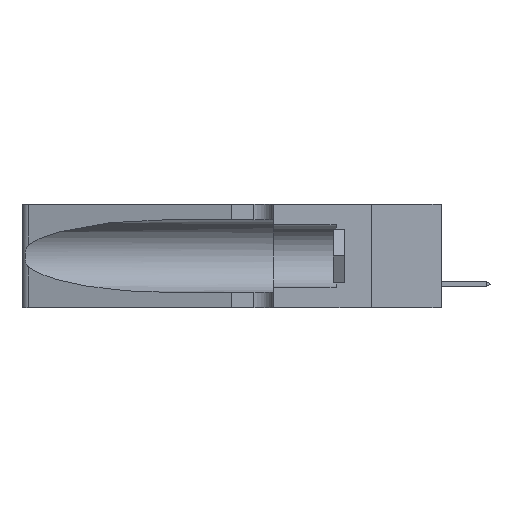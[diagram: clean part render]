
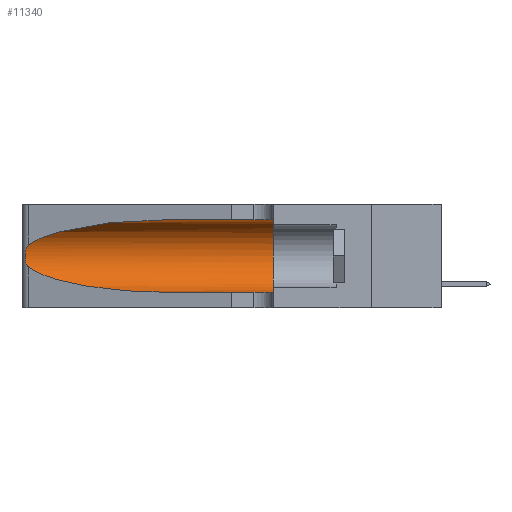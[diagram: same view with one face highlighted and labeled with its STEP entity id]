
A CAD part, left-side view. The second image highlights one B-rep face of the part: STEP entity #11340.
In plain terms, the highlighted cylindrical face has radius 3.308 mm (diameter 6.617 mm), a partial arc.
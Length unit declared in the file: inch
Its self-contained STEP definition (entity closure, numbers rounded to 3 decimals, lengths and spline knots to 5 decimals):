
#604 = EDGE_CURVE ( 'NONE', #4491, #828, #35944, .T. ) ;
#828 = VERTEX_POINT ( 'NONE', #34601 ) ;
#1053 = DIRECTION ( 'NONE',  ( 0., 0., 1. ) ) ;
#1105 = DIRECTION ( 'NONE',  ( 0., -1., 0. ) ) ;
#1410 = CARTESIAN_POINT ( 'NONE',  ( 0.1305, 0.35, 0.31525 ) ) ;
#1831 = CARTESIAN_POINT ( 'NONE',  ( 0.25487, 1.22718, 0.22369 ) ) ;
#1986 = CARTESIAN_POINT ( 'NONE',  ( 0.2373, 1.15595, 0.08982 ) ) ;
#2128 = ORIENTED_EDGE ( 'NONE', *, *, #12219, .F. ) ;
#2251 = EDGE_LOOP ( 'NONE', ( #20262, #12538, #23843, #12944, #31784, #2128 ) ) ;
#2801 = VERTEX_POINT ( 'NONE', #34864 ) ;
#3267 = CYLINDRICAL_SURFACE ( 'NONE', #34637, 0.13025 ) ;
#3283 = CARTESIAN_POINT ( 'NONE',  ( 0.25487, 1.22718, 0.22369 ) ) ;
#4491 = VERTEX_POINT ( 'NONE', #1410 ) ;
#4617 = CARTESIAN_POINT ( 'NONE',  ( 0.2373, 1.15595, 0.28018 ) ) ;
#5232 = CARTESIAN_POINT ( 'NONE',  ( 0.25854, 1.2359, 0.20912 ) ) ;
#5369 = EDGE_CURVE ( 'NONE', #37503, #828, #29029, .T. ) ;
#6507 = DIRECTION ( 'NONE',  ( 0., 0., -1. ) ) ;
#7667 = CARTESIAN_POINT ( 'NONE',  ( 0.18966, 0.96281, 0.31525 ) ) ;
#8292 = CARTESIAN_POINT ( 'NONE',  ( 0.26075, 1.23896, 0.19203 ) ) ;
#8536 = CARTESIAN_POINT ( 'NONE',  ( 0.26075, 1.23896, 0.178 ) ) ;
#9191 = CARTESIAN_POINT ( 'NONE',  ( 0.1305, 0.35, 0.185 ) ) ;
#9451 = EDGE_CURVE ( 'NONE', #23113, #15877, #34838, .T. ) ;
#9644 = EDGE_CURVE ( 'NONE', #2801, #23113, #21317, .T. ) ;
#10951 = CARTESIAN_POINT ( 'NONE',  ( 0.25789, 1.23486, 0.15765 ) ) ;
#11340 = ADVANCED_FACE ( 'NONE', ( #36887 ), #3267, .F. ) ;
#11446 = CARTESIAN_POINT ( 'NONE',  ( 0.26017, 1.23833, 0.17102 ) ) ;
#12211 = DIRECTION ( 'NONE',  ( 0., 1., 0. ) ) ;
#12219 = EDGE_CURVE ( 'NONE', #2801, #4491, #19035, .T. ) ;
#12538 = ORIENTED_EDGE ( 'NONE', *, *, #9451, .T. ) ;
#12944 = ORIENTED_EDGE ( 'NONE', *, *, #5369, .T. ) ;
#13208 = CARTESIAN_POINT ( 'NONE',  ( 0.1305, 0.72297, 0.05475 ) ) ;
#15877 = VERTEX_POINT ( 'NONE', #16320 ) ;
#16320 = CARTESIAN_POINT ( 'NONE',  ( 0.25487, 1.22718, 0.14631 ) ) ;
#16535 = CARTESIAN_POINT ( 'NONE',  ( 0.1305, 0.72297, 0.05475 ) ) ;
#16763 = CARTESIAN_POINT ( 'NONE',  ( 0.25487, 1.22718, 0.14631 ) ) ;
#19035 = LINE ( 'NONE', #32885, #25435 ) ;
#19750 = CARTESIAN_POINT ( 'NONE',  ( 0.25487, 1.22718, 0.22369 ) ) ;
#20262 = ORIENTED_EDGE ( 'NONE', *, *, #9644, .T. ) ;
#21317 =( BOUNDED_CURVE ( )  B_SPLINE_CURVE ( 3, ( #36551, #7667, #4617, #1831 ),
 .UNSPECIFIED., .F., .T. ) 
 B_SPLINE_CURVE_WITH_KNOTS ( ( 4, 4 ),
 ( 1.5708, 2.84003 ),
 .UNSPECIFIED. ) 
 CURVE ( )  GEOMETRIC_REPRESENTATION_ITEM ( )  RATIONAL_B_SPLINE_CURVE ( ( 1., 0.87, 0.87, 1. ) ) 
 REPRESENTATION_ITEM ( '' )  );
#22098 = CARTESIAN_POINT ( 'NONE',  ( 0.18966, 0.96281, 0.05475 ) ) ;
#22567 = CARTESIAN_POINT ( 'NONE',  ( 0.25639, 1.23184, 0.21858 ) ) ;
#22701 = CARTESIAN_POINT ( 'NONE',  ( 0.25555, 1.22994, 0.2215 ) ) ;
#23113 = VERTEX_POINT ( 'NONE', #3283 ) ;
#23625 =( BOUNDED_CURVE ( )  B_SPLINE_CURVE ( 3, ( #24885, #1986, #22098, #16535 ),
 .UNSPECIFIED., .F., .T. ) 
 B_SPLINE_CURVE_WITH_KNOTS ( ( 4, 4 ),
 ( 3.44316, 4.71239 ),
 .UNSPECIFIED. ) 
 CURVE ( )  GEOMETRIC_REPRESENTATION_ITEM ( )  RATIONAL_B_SPLINE_CURVE ( ( 1., 0.87, 0.87, 1. ) ) 
 REPRESENTATION_ITEM ( '' )  );
#23843 = ORIENTED_EDGE ( 'NONE', *, *, #30488, .T. ) ;
#24885 = CARTESIAN_POINT ( 'NONE',  ( 0.25487, 1.22718, 0.14631 ) ) ;
#25435 = VECTOR ( 'NONE', #1105, 39.37008 ) ;
#25591 = CARTESIAN_POINT ( 'NONE',  ( 0.25787, 1.23484, 0.2124 ) ) ;
#25872 = VECTOR ( 'NONE', #28149, 39.37008 ) ;
#25971 = CARTESIAN_POINT ( 'NONE',  ( 0.1305, 1.61858, 0.185 ) ) ;
#28149 = DIRECTION ( 'NONE',  ( 0., -1., 0. ) ) ;
#29029 = LINE ( 'NONE', #37041, #25872 ) ;
#29122 = AXIS2_PLACEMENT_3D ( 'NONE', #9191, #12211, #1053 ) ;
#29362 = DIRECTION ( 'NONE',  ( 0., -1., 0. ) ) ;
#30488 = EDGE_CURVE ( 'NONE', #15877, #37503, #23625, .T. ) ;
#31175 = CARTESIAN_POINT ( 'NONE',  ( 0.25555, 1.22993, 0.14849 ) ) ;
#31552 = CARTESIAN_POINT ( 'NONE',  ( 0.26018, 1.23835, 0.19895 ) ) ;
#31687 = CARTESIAN_POINT ( 'NONE',  ( 0.25639, 1.23186, 0.15144 ) ) ;
#31784 = ORIENTED_EDGE ( 'NONE', *, *, #604, .F. ) ;
#32885 = CARTESIAN_POINT ( 'NONE',  ( 0.1305, 1.61858, 0.31525 ) ) ;
#34113 = CARTESIAN_POINT ( 'NONE',  ( 0.25856, 1.23593, 0.16098 ) ) ;
#34601 = CARTESIAN_POINT ( 'NONE',  ( 0.1305, 0.35, 0.05475 ) ) ;
#34637 = AXIS2_PLACEMENT_3D ( 'NONE', #25971, #29362, #6507 ) ;
#34838 = B_SPLINE_CURVE_WITH_KNOTS ( 'NONE', 3,
 ( #19750, #22701, #22567, #25591, #5232, #31552, #8292, #8536, #11446, #34113, #10951, #31687, #31175, #16763 ),
 .UNSPECIFIED., .F., .F.,
 ( 4, 2, 2, 2, 2, 2, 4 ),
 ( 0., 0.00027, 0.00053, 0.00107, 0.0016, 0.00187, 0.00214 ),
 .UNSPECIFIED. ) ;
#34864 = CARTESIAN_POINT ( 'NONE',  ( 0.1305, 0.72297, 0.31525 ) ) ;
#35944 = CIRCLE ( 'NONE', #29122, 0.13025 ) ;
#36551 = CARTESIAN_POINT ( 'NONE',  ( 0.1305, 0.72297, 0.31525 ) ) ;
#36887 = FACE_OUTER_BOUND ( 'NONE', #2251, .T. ) ;
#37041 = CARTESIAN_POINT ( 'NONE',  ( 0.1305, 1.61858, 0.05475 ) ) ;
#37503 = VERTEX_POINT ( 'NONE', #13208 ) ;
